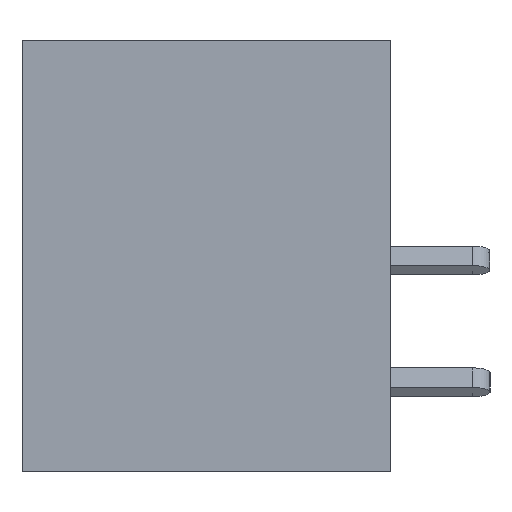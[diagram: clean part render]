
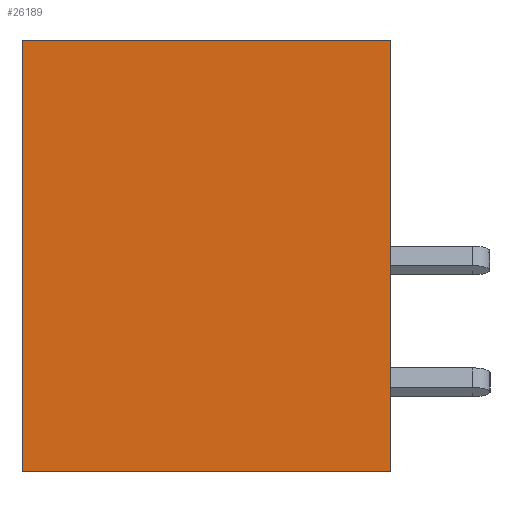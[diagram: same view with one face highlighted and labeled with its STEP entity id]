
A CAD part, left-side view. The second image highlights one B-rep face of the part: STEP entity #26189.
In plain terms, the highlighted planar face has unit normal (-1, 0, 0).
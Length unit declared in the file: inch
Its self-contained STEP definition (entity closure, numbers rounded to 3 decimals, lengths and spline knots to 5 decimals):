
#20 = LINE ( 'NONE', #12075, #1024 ) ;
#34 = EDGE_CURVE ( 'NONE', #22724, #19852, #20, .T. ) ;
#1024 = VECTOR ( 'NONE', #14517, 39.37008 ) ;
#1201 = CARTESIAN_POINT ( 'NONE',  ( 0., 0.453, 0. ) ) ;
#4740 = CARTESIAN_POINT ( 'NONE',  ( 0., 0., -0.531 ) ) ;
#5354 = EDGE_LOOP ( 'NONE', ( #27544, #21579, #14637, #9117 ) ) ;
#6100 = CARTESIAN_POINT ( 'NONE',  ( 0., 0.453, -0.531 ) ) ;
#7639 = CARTESIAN_POINT ( 'NONE',  ( 0., 0.453, -0.531 ) ) ;
#7867 = CARTESIAN_POINT ( 'NONE',  ( 0., 0.453, 0. ) ) ;
#7919 = DIRECTION ( 'NONE',  ( 0., -1., 0. ) ) ;
#8477 = VECTOR ( 'NONE', #23316, 39.37008 ) ;
#9117 = ORIENTED_EDGE ( 'NONE', *, *, #19943, .T. ) ;
#10097 = FACE_OUTER_BOUND ( 'NONE', #5354, .T. ) ;
#11071 = CARTESIAN_POINT ( 'NONE',  ( 0., 0.453, 0. ) ) ;
#11875 = CARTESIAN_POINT ( 'NONE',  ( 0., 0.453, 0. ) ) ;
#12038 = DIRECTION ( 'NONE',  ( 1., 0., 0. ) ) ;
#12075 = CARTESIAN_POINT ( 'NONE',  ( 0., 0., 0. ) ) ;
#12082 = VECTOR ( 'NONE', #7919, 39.37008 ) ;
#12226 = LINE ( 'NONE', #11071, #24330 ) ;
#14392 = PLANE ( 'NONE',  #18659 ) ;
#14517 = DIRECTION ( 'NONE',  ( 0., 0., 1. ) ) ;
#14637 = ORIENTED_EDGE ( 'NONE', *, *, #18338, .F. ) ;
#17814 = LINE ( 'NONE', #7639, #12082 ) ;
#18338 = EDGE_CURVE ( 'NONE', #21834, #18853, #20631, .T. ) ;
#18659 = AXIS2_PLACEMENT_3D ( 'NONE', #7867, #12038, #27249 ) ;
#18853 = VERTEX_POINT ( 'NONE', #11875 ) ;
#19852 = VERTEX_POINT ( 'NONE', #24684 ) ;
#19943 = EDGE_CURVE ( 'NONE', #21834, #22724, #17814, .T. ) ;
#20631 = LINE ( 'NONE', #1201, #8477 ) ;
#21579 = ORIENTED_EDGE ( 'NONE', *, *, #22667, .F. ) ;
#21834 = VERTEX_POINT ( 'NONE', #6100 ) ;
#22667 = EDGE_CURVE ( 'NONE', #18853, #19852, #12226, .T. ) ;
#22724 = VERTEX_POINT ( 'NONE', #4740 ) ;
#23316 = DIRECTION ( 'NONE',  ( 0., 0., 1. ) ) ;
#24330 = VECTOR ( 'NONE', #26271, 39.37008 ) ;
#24684 = CARTESIAN_POINT ( 'NONE',  ( 0., 0., 0. ) ) ;
#26189 = ADVANCED_FACE ( 'NONE', ( #10097 ), #14392, .F. ) ;
#26271 = DIRECTION ( 'NONE',  ( 0., -1., 0. ) ) ;
#27249 = DIRECTION ( 'NONE',  ( 0., 0., -1. ) ) ;
#27544 = ORIENTED_EDGE ( 'NONE', *, *, #34, .T. ) ;
